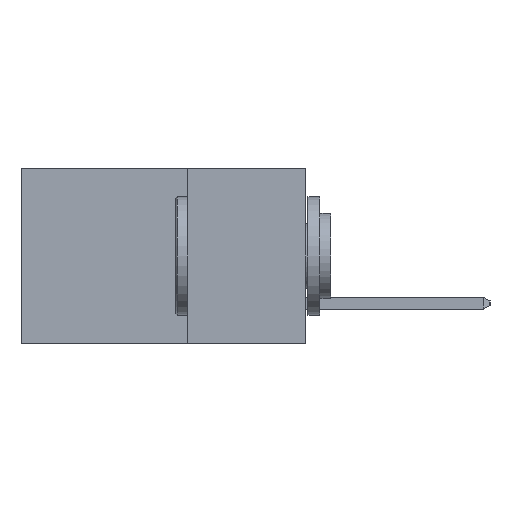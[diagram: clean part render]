
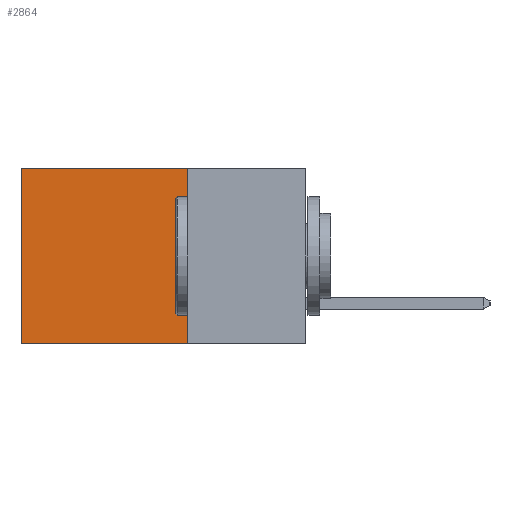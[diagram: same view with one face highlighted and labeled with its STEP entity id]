
A CAD part, left-side view. The second image highlights one B-rep face of the part: STEP entity #2864.
In plain terms, the highlighted planar face has unit normal (-1, 0, 0).
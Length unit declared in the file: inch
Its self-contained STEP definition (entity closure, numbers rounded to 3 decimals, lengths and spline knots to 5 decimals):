
#53 = ORIENTED_EDGE ( 'NONE', *, *, #7857, .T. ) ;
#853 = VERTEX_POINT ( 'NONE', #1207 ) ;
#1207 = CARTESIAN_POINT ( 'NONE',  ( 0.298, 0.25, 0. ) ) ;
#1269 = DIRECTION ( 'NONE',  ( 0., 1., 0. ) ) ;
#1626 = DIRECTION ( 'NONE',  ( 0., 0., -1. ) ) ;
#1658 = EDGE_CURVE ( 'NONE', #12717, #10523, #12852, .T. ) ;
#1990 = VECTOR ( 'NONE', #2167, 39.37008 ) ;
#2167 = DIRECTION ( 'NONE',  ( 0., 1., 0. ) ) ;
#2273 = CARTESIAN_POINT ( 'NONE',  ( 0.298, 0.25, 0. ) ) ;
#2489 = CARTESIAN_POINT ( 'NONE',  ( 0.298, 0.6, 0. ) ) ;
#2528 = FACE_OUTER_BOUND ( 'NONE', #4175, .T. ) ;
#2864 = ADVANCED_FACE ( 'NONE', ( #2528 ), #3016, .F. ) ;
#3016 = PLANE ( 'NONE',  #7825 ) ;
#3619 = CARTESIAN_POINT ( 'NONE',  ( 0.298, 0.25, -0.37 ) ) ;
#3862 = EDGE_CURVE ( 'NONE', #853, #6117, #9132, .T. ) ;
#4175 = EDGE_LOOP ( 'NONE', ( #6971, #6847, #6902, #53 ) ) ;
#5878 = LINE ( 'NONE', #7358, #10965 ) ;
#6065 = CARTESIAN_POINT ( 'NONE',  ( 0.298, 0.6, -0.37 ) ) ;
#6117 = VERTEX_POINT ( 'NONE', #3619 ) ;
#6633 = VECTOR ( 'NONE', #7779, 39.37008 ) ;
#6847 = ORIENTED_EDGE ( 'NONE', *, *, #9512, .F. ) ;
#6890 = DIRECTION ( 'NONE',  ( 0., 0., -1. ) ) ;
#6902 = ORIENTED_EDGE ( 'NONE', *, *, #3862, .F. ) ;
#6971 = ORIENTED_EDGE ( 'NONE', *, *, #1658, .T. ) ;
#7358 = CARTESIAN_POINT ( 'NONE',  ( 0.298, 0.25, 0. ) ) ;
#7779 = DIRECTION ( 'NONE',  ( 0., 0., -1. ) ) ;
#7803 = VECTOR ( 'NONE', #1626, 39.37008 ) ;
#7825 = AXIS2_PLACEMENT_3D ( 'NONE', #2273, #11408, #6890 ) ;
#7857 = EDGE_CURVE ( 'NONE', #853, #12717, #5878, .T. ) ;
#8659 = CARTESIAN_POINT ( 'NONE',  ( 0.298, 0.25, 0. ) ) ;
#9132 = LINE ( 'NONE', #8659, #6633 ) ;
#9512 = EDGE_CURVE ( 'NONE', #6117, #10523, #9884, .T. ) ;
#9884 = LINE ( 'NONE', #11934, #1990 ) ;
#10523 = VERTEX_POINT ( 'NONE', #6065 ) ;
#10965 = VECTOR ( 'NONE', #1269, 39.37008 ) ;
#11333 = CARTESIAN_POINT ( 'NONE',  ( 0.298, 0.6, 0. ) ) ;
#11408 = DIRECTION ( 'NONE',  ( 1., 0., 0. ) ) ;
#11934 = CARTESIAN_POINT ( 'NONE',  ( 0.298, 0.25, -0.37 ) ) ;
#12717 = VERTEX_POINT ( 'NONE', #2489 ) ;
#12852 = LINE ( 'NONE', #11333, #7803 ) ;
